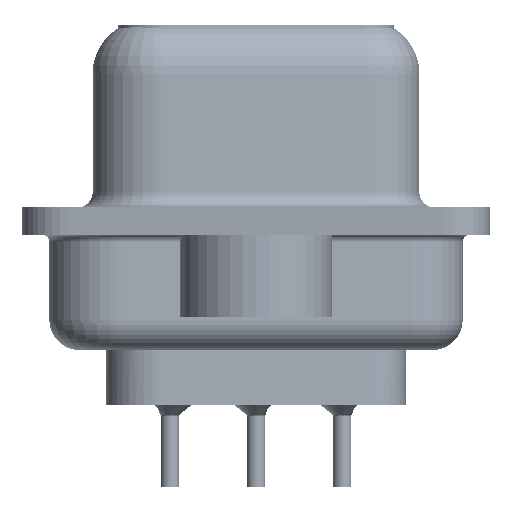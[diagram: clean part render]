
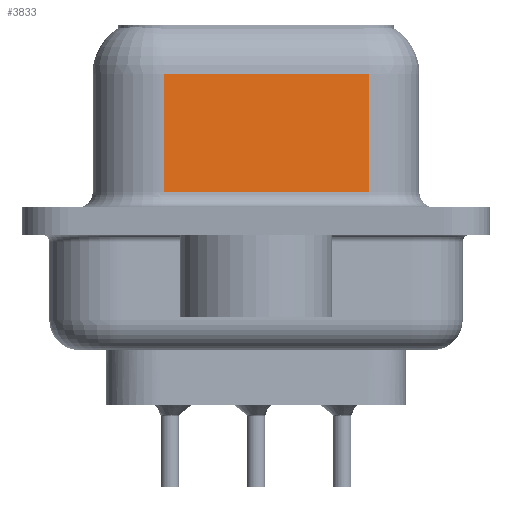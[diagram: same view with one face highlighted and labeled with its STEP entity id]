
A CAD part, left-side view. The second image highlights one B-rep face of the part: STEP entity #3833.
In plain terms, the highlighted planar face has unit normal (-0.985, -0.174, 0).
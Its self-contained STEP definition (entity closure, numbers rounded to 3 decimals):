
#3833 = ADVANCED_FACE ( 'NONE', ( #4178 ), #18383, .F. ) ;
#4178 = FACE_OUTER_BOUND ( 'NONE', #20989, .T. ) ;
#6643 = LINE ( 'NONE', #23434, #39969 ) ;
#6717 = ORIENTED_EDGE ( 'NONE', *, *, #16668, .T. ) ;
#8436 = EDGE_CURVE ( 'NONE', #32800, #14238, #16060, .T. ) ;
#9673 = AXIS2_PLACEMENT_3D ( 'NONE', #18565, #34094, #18330 ) ;
#9919 = CARTESIAN_POINT ( 'NONE',  ( 5.621, -3.722, 0.95 ) ) ;
#11040 = VECTOR ( 'NONE', #39887, 1000. ) ;
#12766 = VERTEX_POINT ( 'NONE', #41056 ) ;
#13198 = CARTESIAN_POINT ( 'NONE',  ( 5.621, -3.722, 4.85 ) ) ;
#13649 = ORIENTED_EDGE ( 'NONE', *, *, #39762, .T. ) ;
#13997 = VECTOR ( 'NONE', #37906, 1000. ) ;
#14238 = VERTEX_POINT ( 'NONE', #21693 ) ;
#16060 = LINE ( 'NONE', #28303, #13997 ) ;
#16591 = CARTESIAN_POINT ( 'NONE',  ( 5.621, -3.722, 6.6 ) ) ;
#16668 = EDGE_CURVE ( 'NONE', #12766, #29936, #6643, .T. ) ;
#17529 = CARTESIAN_POINT ( 'NONE',  ( 4.43, 3.028, 6.6 ) ) ;
#18330 = DIRECTION ( 'NONE',  ( -0.174, 0.985, 0. ) ) ;
#18383 = PLANE ( 'NONE',  #9673 ) ;
#18565 = CARTESIAN_POINT ( 'NONE',  ( 5.621, -3.722, 6.6 ) ) ;
#20989 = EDGE_LOOP ( 'NONE', ( #34988, #41114, #13649, #6717 ) ) ;
#21693 = CARTESIAN_POINT ( 'NONE',  ( 4.43, 3.028, 4.85 ) ) ;
#23434 = CARTESIAN_POINT ( 'NONE',  ( 5.621, -3.722, 0.95 ) ) ;
#25327 = EDGE_CURVE ( 'NONE', #32800, #29936, #40733, .T. ) ;
#28303 = CARTESIAN_POINT ( 'NONE',  ( 5.621, -3.722, 4.85 ) ) ;
#29936 = VERTEX_POINT ( 'NONE', #9919 ) ;
#32298 = VECTOR ( 'NONE', #32732, 1000. ) ;
#32732 = DIRECTION ( 'NONE',  ( 0., 0., -1. ) ) ;
#32800 = VERTEX_POINT ( 'NONE', #13198 ) ;
#34094 = DIRECTION ( 'NONE',  ( 0.985, 0.174, 0. ) ) ;
#34988 = ORIENTED_EDGE ( 'NONE', *, *, #25327, .F. ) ;
#35769 = LINE ( 'NONE', #17529, #11040 ) ;
#37906 = DIRECTION ( 'NONE',  ( -0.174, 0.985, 0. ) ) ;
#39307 = DIRECTION ( 'NONE',  ( 0.174, -0.985, 0. ) ) ;
#39762 = EDGE_CURVE ( 'NONE', #14238, #12766, #35769, .T. ) ;
#39887 = DIRECTION ( 'NONE',  ( 0., 0., -1. ) ) ;
#39969 = VECTOR ( 'NONE', #39307, 1000. ) ;
#40733 = LINE ( 'NONE', #16591, #32298 ) ;
#41056 = CARTESIAN_POINT ( 'NONE',  ( 4.43, 3.028, 0.95 ) ) ;
#41114 = ORIENTED_EDGE ( 'NONE', *, *, #8436, .T. ) ;
